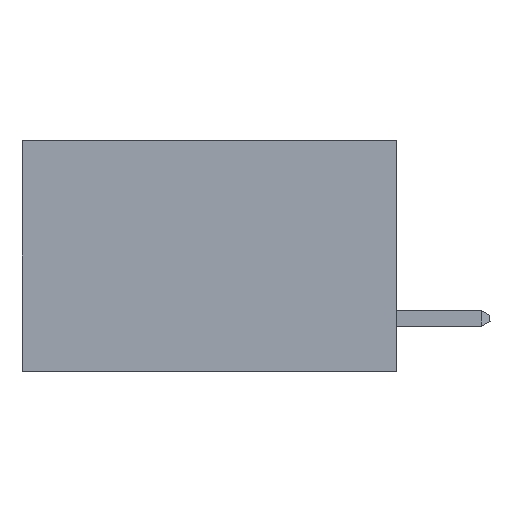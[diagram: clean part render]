
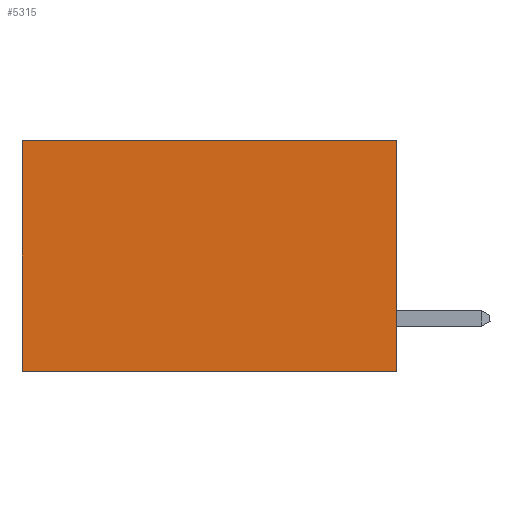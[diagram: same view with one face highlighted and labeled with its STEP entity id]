
A CAD part, left-side view. The second image highlights one B-rep face of the part: STEP entity #5315.
In plain terms, the highlighted planar face has unit normal (-1, 0, 0).
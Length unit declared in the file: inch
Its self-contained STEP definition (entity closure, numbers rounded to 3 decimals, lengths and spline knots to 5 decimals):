
#142 = DIRECTION ( 'NONE',  ( 1., 0., 0. ) ) ;
#159 = CARTESIAN_POINT ( 'NONE',  ( 0.298, 0.6, 0. ) ) ;
#175 = DIRECTION ( 'NONE',  ( 0., 0., -1. ) ) ;
#471 = EDGE_LOOP ( 'NONE', ( #3721, #4162, #3083, #5442 ) ) ;
#625 = VECTOR ( 'NONE', #175, 39.37008 ) ;
#699 = VECTOR ( 'NONE', #10625, 39.37008 ) ;
#705 = CARTESIAN_POINT ( 'NONE',  ( 0.298, 0., -0.37 ) ) ;
#925 = EDGE_CURVE ( 'NONE', #5146, #5728, #9208, .T. ) ;
#1063 = EDGE_CURVE ( 'NONE', #3766, #5728, #5449, .T. ) ;
#1328 = AXIS2_PLACEMENT_3D ( 'NONE', #11171, #142, #10171 ) ;
#1615 = CARTESIAN_POINT ( 'NONE',  ( 0.298, 0.6, 0. ) ) ;
#1980 = PLANE ( 'NONE',  #1328 ) ;
#1998 = CARTESIAN_POINT ( 'NONE',  ( 0.298, 0., 0. ) ) ;
#2431 = VECTOR ( 'NONE', #2538, 39.37008 ) ;
#2538 = DIRECTION ( 'NONE',  ( 0., 0., -1. ) ) ;
#3083 = ORIENTED_EDGE ( 'NONE', *, *, #10225, .F. ) ;
#3248 = CARTESIAN_POINT ( 'NONE',  ( 0.298, 0., -0.37 ) ) ;
#3428 = DIRECTION ( 'NONE',  ( 0., 1., 0. ) ) ;
#3721 = ORIENTED_EDGE ( 'NONE', *, *, #1063, .T. ) ;
#3766 = VERTEX_POINT ( 'NONE', #159 ) ;
#4162 = ORIENTED_EDGE ( 'NONE', *, *, #925, .F. ) ;
#4595 = VECTOR ( 'NONE', #3428, 39.37008 ) ;
#4793 = LINE ( 'NONE', #6617, #625 ) ;
#5146 = VERTEX_POINT ( 'NONE', #705 ) ;
#5315 = ADVANCED_FACE ( 'NONE', ( #6649 ), #1980, .F. ) ;
#5442 = ORIENTED_EDGE ( 'NONE', *, *, #6855, .T. ) ;
#5449 = LINE ( 'NONE', #1615, #2431 ) ;
#5728 = VERTEX_POINT ( 'NONE', #9094 ) ;
#6617 = CARTESIAN_POINT ( 'NONE',  ( 0.298, 0., 0. ) ) ;
#6649 = FACE_OUTER_BOUND ( 'NONE', #471, .T. ) ;
#6855 = EDGE_CURVE ( 'NONE', #7270, #3766, #7496, .T. ) ;
#7270 = VERTEX_POINT ( 'NONE', #1998 ) ;
#7496 = LINE ( 'NONE', #8950, #4595 ) ;
#8950 = CARTESIAN_POINT ( 'NONE',  ( 0.298, 0., 0. ) ) ;
#9094 = CARTESIAN_POINT ( 'NONE',  ( 0.298, 0.6, -0.37 ) ) ;
#9208 = LINE ( 'NONE', #3248, #699 ) ;
#10171 = DIRECTION ( 'NONE',  ( 0., 0., -1. ) ) ;
#10225 = EDGE_CURVE ( 'NONE', #7270, #5146, #4793, .T. ) ;
#10625 = DIRECTION ( 'NONE',  ( 0., 1., 0. ) ) ;
#11171 = CARTESIAN_POINT ( 'NONE',  ( 0.298, 0., 0. ) ) ;
